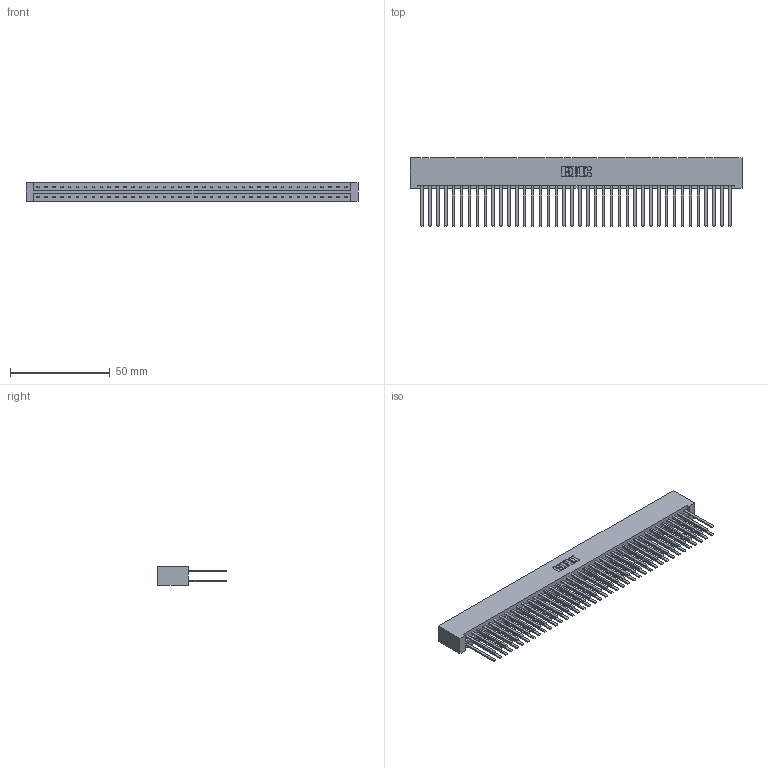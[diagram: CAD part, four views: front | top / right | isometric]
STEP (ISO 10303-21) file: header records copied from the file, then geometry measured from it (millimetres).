
FILE_DESCRIPTION (( 'STEP AP203' ), '1' );
FILE_NAME ('833-080-544-201.STEP', '2020-06-05T22:05:22', ( '' ), ( '' ), 'SwSTEP 2.0', 'SolidWorks 2020', '' );
FILE_SCHEMA (( 'CONFIG_CONTROL_DESIGN' ));
Length unit declared in the file: inch
Products named in the file (3): 833-080-544-201; 345-292-001_345-293-144; 833 Part_Lugless
Assembly tree (81 placements, depth 2):
  833-080-544-201
    833 Part_Lugless
    345-292-001_345-293-144  x80
Bounding box: 166.75 x 34.3 x 9.4 mm (x, y, z)
Volume: 18759.3 mm3; surface area: 25791.8 mm2
Topology: 81 solids, 81 shells, 3786 faces, 11247 edges, 7390 vertices
Faces by surface type: plane 2626, cylinder 1160
Entity records: 25531 total; most frequent: CARTESIAN_POINT 4230, ORIENTED_EDGE 4166, DIRECTION 3607, EDGE_CURVE 2083, LINE 1967, VECTOR 1967, VERTEX_POINT 1386, AXIS2_PLACEMENT_3D 820
